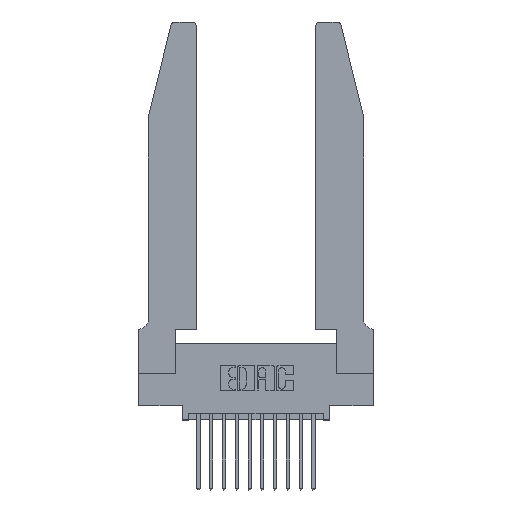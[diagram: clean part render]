
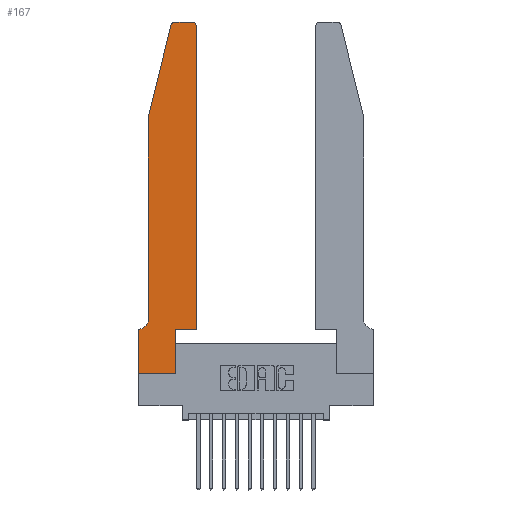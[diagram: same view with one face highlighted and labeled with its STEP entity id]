
A CAD part, top view. The second image highlights one B-rep face of the part: STEP entity #167.
In plain terms, the highlighted planar face has unit normal (0, 0, 1).
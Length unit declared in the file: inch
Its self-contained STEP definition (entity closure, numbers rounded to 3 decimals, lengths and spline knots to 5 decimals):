
#45 = LINE ( 'NONE', #16764, #9771 ) ;
#50 = PLANE ( 'NONE',  #7949 ) ;
#167 = ADVANCED_FACE ( 'NONE', ( #14223 ), #50, .T. ) ;
#340 = DIRECTION ( 'NONE',  ( 0., -1., 0. ) ) ;
#379 = DIRECTION ( 'NONE',  ( -1., 0., 0. ) ) ;
#1057 = VERTEX_POINT ( 'NONE', #2173 ) ;
#1089 = DIRECTION ( 'NONE',  ( 1., 0., 0. ) ) ;
#1485 = VECTOR ( 'NONE', #12110, 39.37008 ) ;
#1708 = EDGE_CURVE ( 'NONE', #11238, #10438, #14985, .T. ) ;
#1914 = VERTEX_POINT ( 'NONE', #5850 ) ;
#2173 = CARTESIAN_POINT ( 'NONE',  ( 0., 0., 0.37 ) ) ;
#2339 = CARTESIAN_POINT ( 'NONE',  ( 0.0055, 0.35, 0.37 ) ) ;
#2460 = CIRCLE ( 'NONE', #12885, 0.03 ) ;
#2897 = CARTESIAN_POINT ( 'NONE',  ( 0.4505, 0.35, 0.37 ) ) ;
#3037 = VERTEX_POINT ( 'NONE', #11827 ) ;
#3082 = VERTEX_POINT ( 'NONE', #2339 ) ;
#3093 = ORIENTED_EDGE ( 'NONE', *, *, #10362, .T. ) ;
#3155 = CIRCLE ( 'NONE', #3549, 0.03 ) ;
#3158 = VECTOR ( 'NONE', #340, 39.37008 ) ;
#3353 = AXIS2_PLACEMENT_3D ( 'NONE', #11071, #9406, #7023 ) ;
#3549 = AXIS2_PLACEMENT_3D ( 'NONE', #7258, #7070, #1089 ) ;
#4098 = EDGE_CURVE ( 'NONE', #7501, #12786, #3155, .T. ) ;
#4152 = EDGE_CURVE ( 'NONE', #13378, #1914, #45, .T. ) ;
#4180 = CARTESIAN_POINT ( 'NONE',  ( 0.4505, 0.35, 0.37 ) ) ;
#4183 = ORIENTED_EDGE ( 'NONE', *, *, #1708, .T. ) ;
#4277 = CARTESIAN_POINT ( 'NONE',  ( 0.284, 2.72, 0.37 ) ) ;
#4434 = LINE ( 'NONE', #14800, #3158 ) ;
#4731 = LINE ( 'NONE', #2897, #13980 ) ;
#4771 = CARTESIAN_POINT ( 'NONE',  ( 0.25487, 2.72718, 0.37 ) ) ;
#4807 = ORIENTED_EDGE ( 'NONE', *, *, #14426, .T. ) ;
#4978 = LINE ( 'NONE', #13161, #6632 ) ;
#5125 = ORIENTED_EDGE ( 'NONE', *, *, #10988, .T. ) ;
#5130 = CARTESIAN_POINT ( 'NONE',  ( 0.4505, 2.72, 0.37 ) ) ;
#5169 = VECTOR ( 'NONE', #14505, 39.37008 ) ;
#5358 = CARTESIAN_POINT ( 'NONE',  ( 0., 0.35, 0.37 ) ) ;
#5850 = CARTESIAN_POINT ( 'NONE',  ( 0.0755, 0.42, 0.37 ) ) ;
#6088 = CARTESIAN_POINT ( 'NONE',  ( 0.4205, 2.75, 0.37 ) ) ;
#6561 = DIRECTION ( 'NONE',  ( 0., 0., 1. ) ) ;
#6606 = EDGE_CURVE ( 'NONE', #11178, #7501, #4731, .T. ) ;
#6609 = DIRECTION ( 'NONE',  ( -0.239, -0.971, 0. ) ) ;
#6632 = VECTOR ( 'NONE', #6609, 39.37008 ) ;
#6914 = ORIENTED_EDGE ( 'NONE', *, *, #13331, .T. ) ;
#7023 = DIRECTION ( 'NONE',  ( -1., 0., 0. ) ) ;
#7070 = DIRECTION ( 'NONE',  ( 0., 0., 1. ) ) ;
#7237 = VERTEX_POINT ( 'NONE', #4771 ) ;
#7258 = CARTESIAN_POINT ( 'NONE',  ( 0.4205, 2.72, 0.37 ) ) ;
#7305 = LINE ( 'NONE', #16132, #1485 ) ;
#7417 = VECTOR ( 'NONE', #17006, 39.37008 ) ;
#7501 = VERTEX_POINT ( 'NONE', #5130 ) ;
#7664 = LINE ( 'NONE', #4180, #5169 ) ;
#7904 = ORIENTED_EDGE ( 'NONE', *, *, #13761, .T. ) ;
#7949 = AXIS2_PLACEMENT_3D ( 'NONE', #5358, #6561, #11802 ) ;
#8253 = DIRECTION ( 'NONE',  ( 0., 1., 0. ) ) ;
#8500 = CARTESIAN_POINT ( 'NONE',  ( 0.284, 2.75, 0.37 ) ) ;
#8560 = CARTESIAN_POINT ( 'NONE',  ( 0.4505, 0.35, 0.37 ) ) ;
#8809 = ORIENTED_EDGE ( 'NONE', *, *, #4152, .T. ) ;
#9034 = ORIENTED_EDGE ( 'NONE', *, *, #10427, .T. ) ;
#9328 = VECTOR ( 'NONE', #13214, 39.37008 ) ;
#9406 = DIRECTION ( 'NONE',  ( 0., 0., -1. ) ) ;
#9771 = VECTOR ( 'NONE', #15737, 39.37008 ) ;
#9919 = EDGE_CURVE ( 'NONE', #3037, #1057, #4434, .T. ) ;
#10362 = EDGE_CURVE ( 'NONE', #1914, #3082, #11014, .T. ) ;
#10427 = EDGE_CURVE ( 'NONE', #1057, #11238, #7305, .T. ) ;
#10438 = VERTEX_POINT ( 'NONE', #13354 ) ;
#10938 = CARTESIAN_POINT ( 'NONE',  ( 0.0755, 2., 0.37 ) ) ;
#10988 = EDGE_CURVE ( 'NONE', #12786, #16485, #13449, .T. ) ;
#11014 = CIRCLE ( 'NONE', #3353, 0.07 ) ;
#11071 = CARTESIAN_POINT ( 'NONE',  ( 0.0055, 0.42, 0.37 ) ) ;
#11178 = VERTEX_POINT ( 'NONE', #8560 ) ;
#11238 = VERTEX_POINT ( 'NONE', #13831 ) ;
#11802 = DIRECTION ( 'NONE',  ( 1., 0., 0. ) ) ;
#11821 = VECTOR ( 'NONE', #379, 39.37008 ) ;
#11827 = CARTESIAN_POINT ( 'NONE',  ( 0., 0.35, 0.37 ) ) ;
#12110 = DIRECTION ( 'NONE',  ( 1., 0., 0. ) ) ;
#12260 = ORIENTED_EDGE ( 'NONE', *, *, #6606, .T. ) ;
#12360 = ORIENTED_EDGE ( 'NONE', *, *, #9919, .T. ) ;
#12368 = ORIENTED_EDGE ( 'NONE', *, *, #12685, .T. ) ;
#12685 = EDGE_CURVE ( 'NONE', #3082, #3037, #13051, .T. ) ;
#12786 = VERTEX_POINT ( 'NONE', #6088 ) ;
#12885 = AXIS2_PLACEMENT_3D ( 'NONE', #4277, #13470, #16077 ) ;
#13051 = LINE ( 'NONE', #16099, #11821 ) ;
#13161 = CARTESIAN_POINT ( 'NONE',  ( 0.0755, 2., 0.37 ) ) ;
#13214 = DIRECTION ( 'NONE',  ( -1., 0., 0. ) ) ;
#13331 = EDGE_CURVE ( 'NONE', #16485, #7237, #2460, .T. ) ;
#13354 = CARTESIAN_POINT ( 'NONE',  ( 0.2865, 0.35, 0.37 ) ) ;
#13378 = VERTEX_POINT ( 'NONE', #10938 ) ;
#13449 = LINE ( 'NONE', #15891, #9328 ) ;
#13470 = DIRECTION ( 'NONE',  ( 0., 0., 1. ) ) ;
#13761 = EDGE_CURVE ( 'NONE', #7237, #13378, #4978, .T. ) ;
#13831 = CARTESIAN_POINT ( 'NONE',  ( 0.2865, 0., 0.37 ) ) ;
#13980 = VECTOR ( 'NONE', #8253, 39.37008 ) ;
#14223 = FACE_OUTER_BOUND ( 'NONE', #15319, .T. ) ;
#14426 = EDGE_CURVE ( 'NONE', #10438, #11178, #7664, .T. ) ;
#14505 = DIRECTION ( 'NONE',  ( 1., 0., 0. ) ) ;
#14800 = CARTESIAN_POINT ( 'NONE',  ( 0., 0., 0.37 ) ) ;
#14985 = LINE ( 'NONE', #15525, #7417 ) ;
#15319 = EDGE_LOOP ( 'NONE', ( #5125, #6914, #7904, #8809, #3093, #12368, #12360, #9034, #4183, #4807, #12260, #15581 ) ) ;
#15525 = CARTESIAN_POINT ( 'NONE',  ( 0.2865, 0.35, 0.37 ) ) ;
#15581 = ORIENTED_EDGE ( 'NONE', *, *, #4098, .T. ) ;
#15737 = DIRECTION ( 'NONE',  ( 0., -1., 0. ) ) ;
#15891 = CARTESIAN_POINT ( 'NONE',  ( 0.2605, 2.75, 0.37 ) ) ;
#16077 = DIRECTION ( 'NONE',  ( 1., 0., 0. ) ) ;
#16099 = CARTESIAN_POINT ( 'NONE',  ( 0.0755, 0.35, 0.37 ) ) ;
#16132 = CARTESIAN_POINT ( 'NONE',  ( 0., 0., 0.37 ) ) ;
#16485 = VERTEX_POINT ( 'NONE', #8500 ) ;
#16764 = CARTESIAN_POINT ( 'NONE',  ( 0.0755, 2., 0.37 ) ) ;
#17006 = DIRECTION ( 'NONE',  ( 0., 1., 0. ) ) ;
